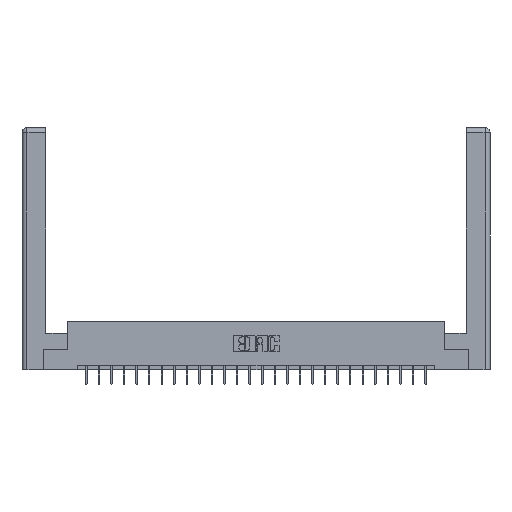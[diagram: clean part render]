
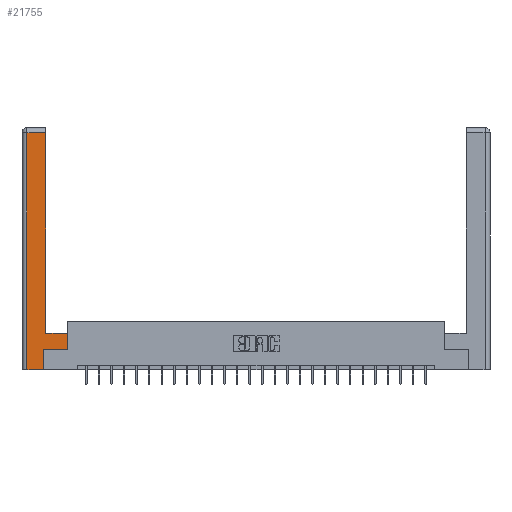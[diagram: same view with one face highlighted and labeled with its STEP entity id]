
A CAD part, top view. The second image highlights one B-rep face of the part: STEP entity #21755.
In plain terms, the highlighted planar face has unit normal (0, 0, 1).
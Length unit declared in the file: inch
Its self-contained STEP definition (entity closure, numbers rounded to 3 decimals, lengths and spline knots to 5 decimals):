
#187 = LINE ( 'NONE', #25757, #2066 ) ;
#648 = LINE ( 'NONE', #14031, #8568 ) ;
#1003 = LINE ( 'NONE', #22005, #11750 ) ;
#1257 = DIRECTION ( 'NONE',  ( 0., -1., 0. ) ) ;
#1332 = VECTOR ( 'NONE', #14181, 39.37008 ) ;
#1348 = CARTESIAN_POINT ( 'NONE',  ( 0.295, 0.45, 0. ) ) ;
#1410 = DIRECTION ( 'NONE',  ( 0., 1., 0. ) ) ;
#1848 = VERTEX_POINT ( 'NONE', #4027 ) ;
#2066 = VECTOR ( 'NONE', #1257, 39.37008 ) ;
#2547 = PLANE ( 'NONE',  #3406 ) ;
#3406 = AXIS2_PLACEMENT_3D ( 'NONE', #20823, #24512, #12653 ) ;
#3442 = EDGE_CURVE ( 'NONE', #19393, #8434, #648, .T. ) ;
#3614 = ORIENTED_EDGE ( 'NONE', *, *, #21232, .T. ) ;
#3799 = CARTESIAN_POINT ( 'NONE',  ( 0.295, 2.94, 0. ) ) ;
#4027 = CARTESIAN_POINT ( 'NONE',  ( 0.565, 0.45, 0. ) ) ;
#4636 = VERTEX_POINT ( 'NONE', #24866 ) ;
#4917 = DIRECTION ( 'NONE',  ( 1., 0., 0. ) ) ;
#5362 = EDGE_CURVE ( 'NONE', #8434, #14871, #8468, .T. ) ;
#5938 = CARTESIAN_POINT ( 'NONE',  ( 0.295, 0.45, 0. ) ) ;
#6433 = VECTOR ( 'NONE', #4917, 39.37008 ) ;
#6756 = VERTEX_POINT ( 'NONE', #10951 ) ;
#7307 = ORIENTED_EDGE ( 'NONE', *, *, #3442, .T. ) ;
#7463 = EDGE_CURVE ( 'NONE', #4636, #19393, #17154, .T. ) ;
#7709 = DIRECTION ( 'NONE',  ( -1., 0., 0. ) ) ;
#8036 = DIRECTION ( 'NONE',  ( 0., 1., 0. ) ) ;
#8400 = ORIENTED_EDGE ( 'NONE', *, *, #12130, .T. ) ;
#8434 = VERTEX_POINT ( 'NONE', #23724 ) ;
#8468 = LINE ( 'NONE', #10819, #16958 ) ;
#8568 = VECTOR ( 'NONE', #8036, 39.37008 ) ;
#8798 = EDGE_CURVE ( 'NONE', #25762, #13722, #1003, .T. ) ;
#8882 = DIRECTION ( 'NONE',  ( 1., 0., 0. ) ) ;
#9410 = LINE ( 'NONE', #24052, #11907 ) ;
#9695 = VECTOR ( 'NONE', #18707, 39.37008 ) ;
#10350 = ORIENTED_EDGE ( 'NONE', *, *, #5362, .T. ) ;
#10517 = ORIENTED_EDGE ( 'NONE', *, *, #13193, .T. ) ;
#10819 = CARTESIAN_POINT ( 'NONE',  ( 0.565, 0.245, 0. ) ) ;
#10951 = CARTESIAN_POINT ( 'NONE',  ( 0.0615, 2.94, 0. ) ) ;
#11750 = VECTOR ( 'NONE', #1410, 39.37008 ) ;
#11772 = LINE ( 'NONE', #5938, #1332 ) ;
#11907 = VECTOR ( 'NONE', #7709, 39.37008 ) ;
#12130 = EDGE_CURVE ( 'NONE', #13722, #6756, #9410, .T. ) ;
#12653 = DIRECTION ( 'NONE',  ( -1., 0., 0. ) ) ;
#13193 = EDGE_CURVE ( 'NONE', #1848, #25762, #11772, .T. ) ;
#13722 = VERTEX_POINT ( 'NONE', #3799 ) ;
#14031 = CARTESIAN_POINT ( 'NONE',  ( 0.265, 0.245, 0. ) ) ;
#14181 = DIRECTION ( 'NONE',  ( -1., 0., 0. ) ) ;
#14611 = CARTESIAN_POINT ( 'NONE',  ( 0.565, 0.245, 0. ) ) ;
#14708 = FACE_OUTER_BOUND ( 'NONE', #22475, .T. ) ;
#14871 = VERTEX_POINT ( 'NONE', #14611 ) ;
#15033 = CARTESIAN_POINT ( 'NONE',  ( 0.565, 0.45, 0. ) ) ;
#16773 = CARTESIAN_POINT ( 'NONE',  ( 0.265, 0., 0. ) ) ;
#16958 = VECTOR ( 'NONE', #8882, 39.37008 ) ;
#17154 = LINE ( 'NONE', #19001, #6433 ) ;
#17285 = EDGE_CURVE ( 'NONE', #6756, #4636, #187, .T. ) ;
#18707 = DIRECTION ( 'NONE',  ( 0., 1., 0. ) ) ;
#19001 = CARTESIAN_POINT ( 'NONE',  ( 0.265, 0., 0. ) ) ;
#19393 = VERTEX_POINT ( 'NONE', #16773 ) ;
#20397 = LINE ( 'NONE', #15033, #9695 ) ;
#20823 = CARTESIAN_POINT ( 'NONE',  ( 0., 0., 0. ) ) ;
#21232 = EDGE_CURVE ( 'NONE', #14871, #1848, #20397, .T. ) ;
#21755 = ADVANCED_FACE ( 'NONE', ( #14708 ), #2547, .F. ) ;
#22005 = CARTESIAN_POINT ( 'NONE',  ( 0.295, 3., 0. ) ) ;
#22475 = EDGE_LOOP ( 'NONE', ( #25215, #8400, #25214, #23756, #7307, #10350, #3614, #10517 ) ) ;
#23724 = CARTESIAN_POINT ( 'NONE',  ( 0.265, 0.245, 0. ) ) ;
#23756 = ORIENTED_EDGE ( 'NONE', *, *, #7463, .T. ) ;
#24052 = CARTESIAN_POINT ( 'NONE',  ( 0.0615, 2.94, 0. ) ) ;
#24512 = DIRECTION ( 'NONE',  ( 0., 0., -1. ) ) ;
#24866 = CARTESIAN_POINT ( 'NONE',  ( 0.0615, 0., 0. ) ) ;
#25214 = ORIENTED_EDGE ( 'NONE', *, *, #17285, .T. ) ;
#25215 = ORIENTED_EDGE ( 'NONE', *, *, #8798, .T. ) ;
#25757 = CARTESIAN_POINT ( 'NONE',  ( 0.0615, 0., 0. ) ) ;
#25762 = VERTEX_POINT ( 'NONE', #1348 ) ;
